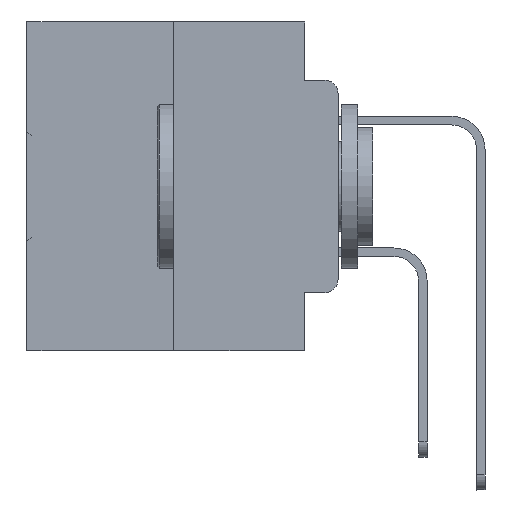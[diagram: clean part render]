
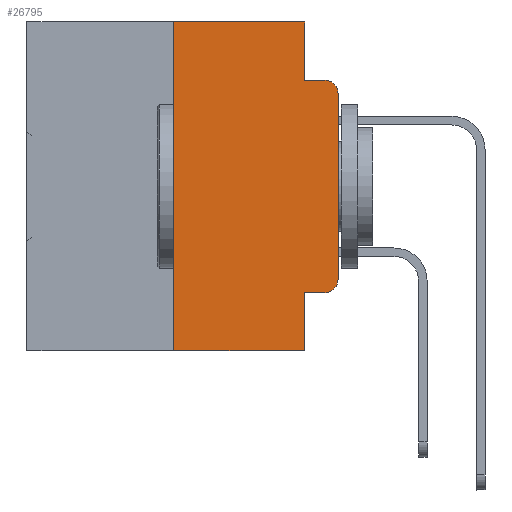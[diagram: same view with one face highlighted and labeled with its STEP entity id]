
A CAD part, left-side view. The second image highlights one B-rep face of the part: STEP entity #26795.
In plain terms, the highlighted planar face has unit normal (-1, 0, 0).
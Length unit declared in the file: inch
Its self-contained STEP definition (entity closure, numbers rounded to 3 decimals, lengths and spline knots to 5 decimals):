
#253 = CIRCLE ( 'NONE', #36305, 0.02 ) ;
#929 = DIRECTION ( 'NONE',  ( 0., -1., 0. ) ) ;
#1030 = VERTEX_POINT ( 'NONE', #20345 ) ;
#1204 = VERTEX_POINT ( 'NONE', #29659 ) ;
#1441 = DIRECTION ( 'NONE',  ( 0., 0., -1. ) ) ;
#2472 = ORIENTED_EDGE ( 'NONE', *, *, #30155, .F. ) ;
#4236 = EDGE_CURVE ( 'NONE', #1204, #12170, #33944, .T. ) ;
#4708 = ORIENTED_EDGE ( 'NONE', *, *, #7871, .T. ) ;
#5467 = CARTESIAN_POINT ( 'NONE',  ( 0., 0.25, 0. ) ) ;
#6602 = CARTESIAN_POINT ( 'NONE',  ( 0., 0.473, 0. ) ) ;
#6876 = CARTESIAN_POINT ( 'NONE',  ( 0., 0., -0.1085 ) ) ;
#7218 = LINE ( 'NONE', #14713, #13921 ) ;
#7820 = VERTEX_POINT ( 'NONE', #5467 ) ;
#7871 = EDGE_CURVE ( 'NONE', #33273, #24955, #35016, .T. ) ;
#7912 = CARTESIAN_POINT ( 'NONE',  ( 0., 0.051, -0.0885 ) ) ;
#7986 = CARTESIAN_POINT ( 'NONE',  ( 0., 0.051, -0.5 ) ) ;
#8582 = ORIENTED_EDGE ( 'NONE', *, *, #18222, .F. ) ;
#8656 = VECTOR ( 'NONE', #34339, 39.37008 ) ;
#8728 = EDGE_CURVE ( 'NONE', #33273, #7820, #18315, .T. ) ;
#8776 = DIRECTION ( 'NONE',  ( -1., 0., 0. ) ) ;
#10123 = VECTOR ( 'NONE', #1441, 39.37008 ) ;
#11270 = ORIENTED_EDGE ( 'NONE', *, *, #22596, .F. ) ;
#12170 = VERTEX_POINT ( 'NONE', #6876 ) ;
#12327 = CARTESIAN_POINT ( 'NONE',  ( 0., 0.02, -0.3915 ) ) ;
#12838 = CARTESIAN_POINT ( 'NONE',  ( 0., 0.051, 0. ) ) ;
#13356 = DIRECTION ( 'NONE',  ( 0., 0., -1. ) ) ;
#13921 = VECTOR ( 'NONE', #34185, 39.37008 ) ;
#14682 = CARTESIAN_POINT ( 'NONE',  ( 0., 0.25, -0.5 ) ) ;
#14713 = CARTESIAN_POINT ( 'NONE',  ( 0., 0.051, -0.0885 ) ) ;
#15151 = DIRECTION ( 'NONE',  ( 0., 0., -1. ) ) ;
#16007 = CARTESIAN_POINT ( 'NONE',  ( 0., 0.25, 0. ) ) ;
#16182 = VERTEX_POINT ( 'NONE', #7912 ) ;
#16436 = VERTEX_POINT ( 'NONE', #34222 ) ;
#16949 = LINE ( 'NONE', #6602, #18692 ) ;
#16967 = ORIENTED_EDGE ( 'NONE', *, *, #4236, .T. ) ;
#16983 = CARTESIAN_POINT ( 'NONE',  ( 0., 0.473, -0.5 ) ) ;
#17440 = VECTOR ( 'NONE', #30063, 39.37008 ) ;
#17559 = DIRECTION ( 'NONE',  ( 0., -1., 0. ) ) ;
#17668 = LINE ( 'NONE', #12838, #10123 ) ;
#18040 = ORIENTED_EDGE ( 'NONE', *, *, #20785, .T. ) ;
#18222 = EDGE_CURVE ( 'NONE', #16436, #16182, #17668, .T. ) ;
#18315 = LINE ( 'NONE', #16007, #17440 ) ;
#18692 = VECTOR ( 'NONE', #929, 39.37008 ) ;
#18877 = ORIENTED_EDGE ( 'NONE', *, *, #8728, .F. ) ;
#18997 = AXIS2_PLACEMENT_3D ( 'NONE', #12327, #31884, #15151 ) ;
#19556 = FACE_OUTER_BOUND ( 'NONE', #24313, .T. ) ;
#20037 = VECTOR ( 'NONE', #23007, 39.37008 ) ;
#20162 = CARTESIAN_POINT ( 'NONE',  ( 0., 0., 0. ) ) ;
#20345 = CARTESIAN_POINT ( 'NONE',  ( 0., 0.02, -0.4115 ) ) ;
#20497 = ORIENTED_EDGE ( 'NONE', *, *, #22005, .F. ) ;
#20785 = EDGE_CURVE ( 'NONE', #1030, #1204, #22794, .T. ) ;
#21718 = CARTESIAN_POINT ( 'NONE',  ( 0., 0.473, 0. ) ) ;
#22005 = EDGE_CURVE ( 'NONE', #16182, #24001, #7218, .T. ) ;
#22596 = EDGE_CURVE ( 'NONE', #7820, #16436, #16949, .T. ) ;
#22794 = CIRCLE ( 'NONE', #18997, 0.02 ) ;
#23007 = DIRECTION ( 'NONE',  ( 0., 0., 1. ) ) ;
#23684 = LINE ( 'NONE', #31589, #8656 ) ;
#23883 = CARTESIAN_POINT ( 'NONE',  ( 0., 0.051, -0.4115 ) ) ;
#24001 = VERTEX_POINT ( 'NONE', #33879 ) ;
#24313 = EDGE_LOOP ( 'NONE', ( #16967, #26625, #20497, #8582, #11270, #18877, #4708, #2472, #34119, #18040 ) ) ;
#24955 = VERTEX_POINT ( 'NONE', #7986 ) ;
#25329 = VERTEX_POINT ( 'NONE', #23883 ) ;
#25686 = CARTESIAN_POINT ( 'NONE',  ( 0., 0.02, -0.1085 ) ) ;
#25749 = EDGE_CURVE ( 'NONE', #12170, #24001, #253, .T. ) ;
#26452 = EDGE_CURVE ( 'NONE', #25329, #1030, #28958, .T. ) ;
#26625 = ORIENTED_EDGE ( 'NONE', *, *, #25749, .T. ) ;
#26795 = ADVANCED_FACE ( 'NONE', ( #19556 ), #29994, .F. ) ;
#28000 = DIRECTION ( 'NONE',  ( 0., -1., 0. ) ) ;
#28483 = DIRECTION ( 'NONE',  ( 0., 0., -1. ) ) ;
#28958 = LINE ( 'NONE', #31466, #35383 ) ;
#29659 = CARTESIAN_POINT ( 'NONE',  ( 0., 0., -0.3915 ) ) ;
#29994 = PLANE ( 'NONE',  #32454 ) ;
#30063 = DIRECTION ( 'NONE',  ( 0., 0., 1. ) ) ;
#30120 = DIRECTION ( 'NONE',  ( 1., 0., 0. ) ) ;
#30155 = EDGE_CURVE ( 'NONE', #25329, #24955, #23684, .T. ) ;
#31466 = CARTESIAN_POINT ( 'NONE',  ( 0., 0.051, -0.4115 ) ) ;
#31589 = CARTESIAN_POINT ( 'NONE',  ( 0., 0.051, 0. ) ) ;
#31884 = DIRECTION ( 'NONE',  ( -1., 0., 0. ) ) ;
#32454 = AXIS2_PLACEMENT_3D ( 'NONE', #21718, #30120, #13356 ) ;
#33273 = VERTEX_POINT ( 'NONE', #14682 ) ;
#33879 = CARTESIAN_POINT ( 'NONE',  ( 0., 0.02, -0.0885 ) ) ;
#33944 = LINE ( 'NONE', #20162, #20037 ) ;
#34119 = ORIENTED_EDGE ( 'NONE', *, *, #26452, .T. ) ;
#34166 = VECTOR ( 'NONE', #28000, 39.37008 ) ;
#34185 = DIRECTION ( 'NONE',  ( 0., -1., 0. ) ) ;
#34222 = CARTESIAN_POINT ( 'NONE',  ( 0., 0.051, 0. ) ) ;
#34339 = DIRECTION ( 'NONE',  ( 0., 0., -1. ) ) ;
#35016 = LINE ( 'NONE', #16983, #34166 ) ;
#35383 = VECTOR ( 'NONE', #17559, 39.37008 ) ;
#36305 = AXIS2_PLACEMENT_3D ( 'NONE', #25686, #8776, #28483 ) ;
